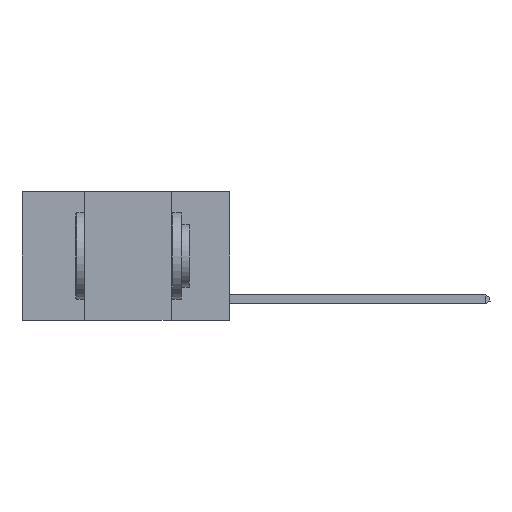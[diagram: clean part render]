
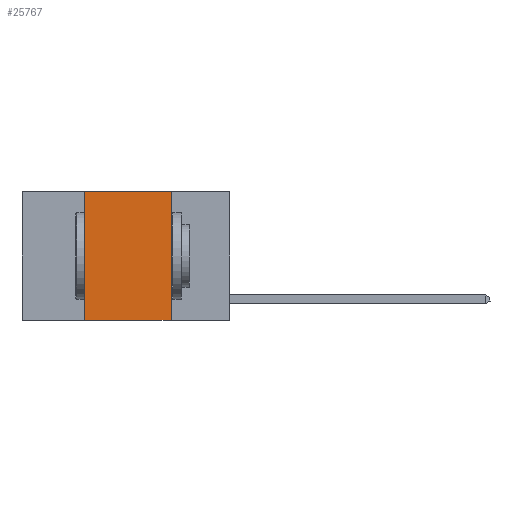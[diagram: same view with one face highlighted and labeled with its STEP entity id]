
A CAD part, left-side view. The second image highlights one B-rep face of the part: STEP entity #25767.
In plain terms, the highlighted planar face has unit normal (-1, 0, 0).
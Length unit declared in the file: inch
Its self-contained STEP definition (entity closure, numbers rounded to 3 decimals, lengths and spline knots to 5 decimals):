
#1538 = PLANE ( 'NONE',  #3191 ) ;
#1880 = DIRECTION ( 'NONE',  ( 0., 0., -1. ) ) ;
#2540 = CARTESIAN_POINT ( 'NONE',  ( 0., 0.42, 0. ) ) ;
#3125 = EDGE_LOOP ( 'NONE', ( #16490, #6463, #24026, #7776 ) ) ;
#3191 = AXIS2_PLACEMENT_3D ( 'NONE', #16055, #8468, #12424 ) ;
#4393 = VERTEX_POINT ( 'NONE', #2540 ) ;
#6463 = ORIENTED_EDGE ( 'NONE', *, *, #7354, .F. ) ;
#7354 = EDGE_CURVE ( 'NONE', #4393, #23962, #8115, .T. ) ;
#7606 = LINE ( 'NONE', #15880, #25386 ) ;
#7776 = ORIENTED_EDGE ( 'NONE', *, *, #13633, .T. ) ;
#8115 = LINE ( 'NONE', #19687, #9703 ) ;
#8297 = VECTOR ( 'NONE', #1880, 39.37008 ) ;
#8468 = DIRECTION ( 'NONE',  ( 1., 0., 0. ) ) ;
#9563 = DIRECTION ( 'NONE',  ( 0., -1., 0. ) ) ;
#9703 = VECTOR ( 'NONE', #23656, 39.37008 ) ;
#11137 = VECTOR ( 'NONE', #11936, 39.37008 ) ;
#11495 = CARTESIAN_POINT ( 'NONE',  ( 0., 0.42, -0.37 ) ) ;
#11844 = VERTEX_POINT ( 'NONE', #11495 ) ;
#11936 = DIRECTION ( 'NONE',  ( 0., 0., 1. ) ) ;
#12366 = EDGE_CURVE ( 'NONE', #23962, #18375, #20922, .T. ) ;
#12424 = DIRECTION ( 'NONE',  ( 0., 0., -1. ) ) ;
#13063 = EDGE_CURVE ( 'NONE', #11844, #4393, #23101, .T. ) ;
#13633 = EDGE_CURVE ( 'NONE', #11844, #18375, #7606, .T. ) ;
#15182 = CARTESIAN_POINT ( 'NONE',  ( 0., 0.17, 0. ) ) ;
#15880 = CARTESIAN_POINT ( 'NONE',  ( 0., 0.6, -0.37 ) ) ;
#16007 = CARTESIAN_POINT ( 'NONE',  ( 0., 0.42, 0. ) ) ;
#16055 = CARTESIAN_POINT ( 'NONE',  ( 0., 0.6, 0. ) ) ;
#16490 = ORIENTED_EDGE ( 'NONE', *, *, #12366, .F. ) ;
#18375 = VERTEX_POINT ( 'NONE', #24978 ) ;
#19687 = CARTESIAN_POINT ( 'NONE',  ( 0., 0.6, 0. ) ) ;
#20733 = CARTESIAN_POINT ( 'NONE',  ( 0., 0.17, 0. ) ) ;
#20922 = LINE ( 'NONE', #20733, #8297 ) ;
#23101 = LINE ( 'NONE', #16007, #11137 ) ;
#23656 = DIRECTION ( 'NONE',  ( 0., -1., 0. ) ) ;
#23962 = VERTEX_POINT ( 'NONE', #15182 ) ;
#24026 = ORIENTED_EDGE ( 'NONE', *, *, #13063, .F. ) ;
#24978 = CARTESIAN_POINT ( 'NONE',  ( 0., 0.17, -0.37 ) ) ;
#25386 = VECTOR ( 'NONE', #9563, 39.37008 ) ;
#25767 = ADVANCED_FACE ( 'NONE', ( #25939 ), #1538, .F. ) ;
#25939 = FACE_OUTER_BOUND ( 'NONE', #3125, .T. ) ;
